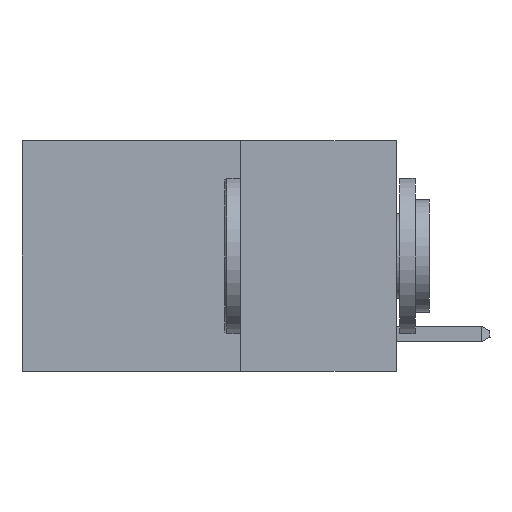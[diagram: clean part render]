
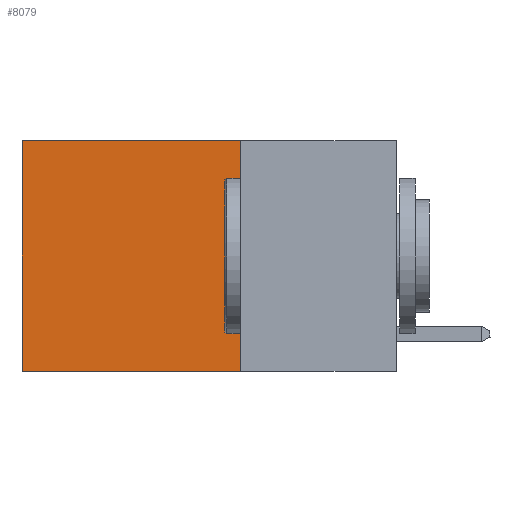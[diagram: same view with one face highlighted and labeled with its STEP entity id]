
A CAD part, left-side view. The second image highlights one B-rep face of the part: STEP entity #8079.
In plain terms, the highlighted planar face has unit normal (-1, 0, 0).
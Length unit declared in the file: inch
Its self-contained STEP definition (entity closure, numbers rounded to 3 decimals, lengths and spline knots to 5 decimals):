
#233 = CARTESIAN_POINT ( 'NONE',  ( 0.2625, 0.6, 0. ) ) ;
#262 = DIRECTION ( 'NONE',  ( 1., 0., 0. ) ) ;
#578 = VECTOR ( 'NONE', #5779, 39.37008 ) ;
#696 = VECTOR ( 'NONE', #16567, 39.37008 ) ;
#1053 = VECTOR ( 'NONE', #8638, 39.37008 ) ;
#2080 = CARTESIAN_POINT ( 'NONE',  ( 0.2625, 0.25, -0.37 ) ) ;
#2694 = ORIENTED_EDGE ( 'NONE', *, *, #10628, .F. ) ;
#2738 = DIRECTION ( 'NONE',  ( 0., 1., 0. ) ) ;
#3525 = EDGE_CURVE ( 'NONE', #12820, #16353, #7776, .T. ) ;
#4151 = EDGE_CURVE ( 'NONE', #12820, #14195, #13244, .T. ) ;
#4620 = LINE ( 'NONE', #15105, #696 ) ;
#5779 = DIRECTION ( 'NONE',  ( 0., 0., -1. ) ) ;
#7188 = CARTESIAN_POINT ( 'NONE',  ( 0.2625, 0.25, 0. ) ) ;
#7204 = EDGE_CURVE ( 'NONE', #16353, #11808, #8423, .T. ) ;
#7776 = LINE ( 'NONE', #17422, #15549 ) ;
#7941 = FACE_OUTER_BOUND ( 'NONE', #14593, .T. ) ;
#8079 = ADVANCED_FACE ( 'NONE', ( #7941 ), #16365, .F. ) ;
#8423 = LINE ( 'NONE', #13083, #578 ) ;
#8638 = DIRECTION ( 'NONE',  ( 0., 0., -1. ) ) ;
#8701 = ORIENTED_EDGE ( 'NONE', *, *, #4151, .F. ) ;
#9086 = CARTESIAN_POINT ( 'NONE',  ( 0.2625, 0.25, 0. ) ) ;
#10560 = DIRECTION ( 'NONE',  ( 0., 0., -1. ) ) ;
#10628 = EDGE_CURVE ( 'NONE', #14195, #11808, #4620, .T. ) ;
#11233 = CARTESIAN_POINT ( 'NONE',  ( 0.2625, 0.25, 0. ) ) ;
#11808 = VERTEX_POINT ( 'NONE', #13286 ) ;
#12820 = VERTEX_POINT ( 'NONE', #11233 ) ;
#13083 = CARTESIAN_POINT ( 'NONE',  ( 0.2625, 0.6, 0. ) ) ;
#13244 = LINE ( 'NONE', #7188, #1053 ) ;
#13286 = CARTESIAN_POINT ( 'NONE',  ( 0.2625, 0.6, -0.37 ) ) ;
#13440 = ORIENTED_EDGE ( 'NONE', *, *, #3525, .T. ) ;
#14195 = VERTEX_POINT ( 'NONE', #2080 ) ;
#14593 = EDGE_LOOP ( 'NONE', ( #16475, #2694, #8701, #13440 ) ) ;
#15105 = CARTESIAN_POINT ( 'NONE',  ( 0.2625, 0.25, -0.37 ) ) ;
#15549 = VECTOR ( 'NONE', #2738, 39.37008 ) ;
#16353 = VERTEX_POINT ( 'NONE', #233 ) ;
#16365 = PLANE ( 'NONE',  #17320 ) ;
#16475 = ORIENTED_EDGE ( 'NONE', *, *, #7204, .T. ) ;
#16567 = DIRECTION ( 'NONE',  ( 0., 1., 0. ) ) ;
#17320 = AXIS2_PLACEMENT_3D ( 'NONE', #9086, #262, #10560 ) ;
#17422 = CARTESIAN_POINT ( 'NONE',  ( 0.2625, 0.25, 0. ) ) ;
